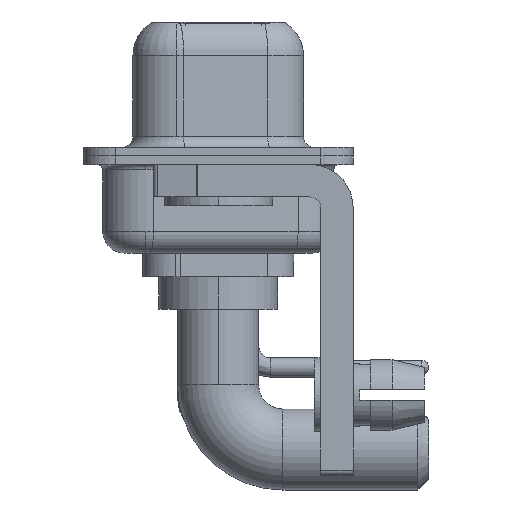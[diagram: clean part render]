
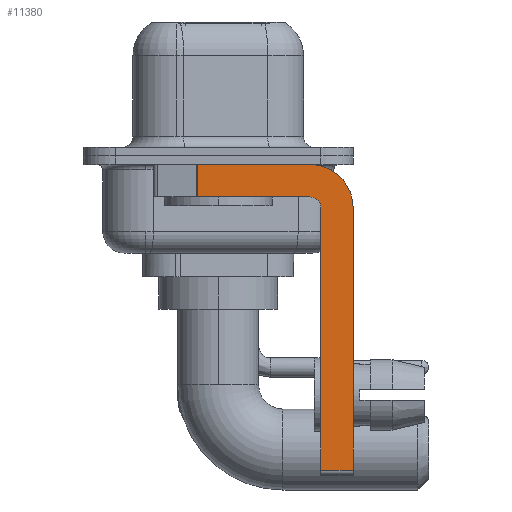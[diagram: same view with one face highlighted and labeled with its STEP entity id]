
A CAD part, left-side view. The second image highlights one B-rep face of the part: STEP entity #11380.
In plain terms, the highlighted planar face has unit normal (-1, 0, 0).
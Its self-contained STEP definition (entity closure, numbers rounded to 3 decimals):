
#782 = EDGE_CURVE ( 'NONE', #16685, #5322, #13096, .T. ) ;
#1770 = VERTEX_POINT ( 'NONE', #12619 ) ;
#1902 = VERTEX_POINT ( 'NONE', #8705 ) ;
#2012 = ORIENTED_EDGE ( 'NONE', *, *, #8583, .F. ) ;
#2090 = AXIS2_PLACEMENT_3D ( 'NONE', #5096, #18434, #12122 ) ;
#2623 = DIRECTION ( 'NONE',  ( 0., 0., -1. ) ) ;
#2792 = CIRCLE ( 'NONE', #18339, 2. ) ;
#2835 = LINE ( 'NONE', #13054, #6087 ) ;
#2849 = ORIENTED_EDGE ( 'NONE', *, *, #8291, .F. ) ;
#2997 = CARTESIAN_POINT ( 'NONE',  ( -2.9, -4.75, -14.8 ) ) ;
#3055 = DIRECTION ( 'NONE',  ( 0., 1., 0. ) ) ;
#3781 = LINE ( 'NONE', #16767, #17156 ) ;
#3980 = LINE ( 'NONE', #8471, #14771 ) ;
#4963 = LINE ( 'NONE', #6529, #10078 ) ;
#5096 = CARTESIAN_POINT ( 'NONE',  ( -2.9, -4.25, -2.4 ) ) ;
#5122 = EDGE_CURVE ( 'NONE', #1902, #5207, #3781, .T. ) ;
#5207 = VERTEX_POINT ( 'NONE', #18219 ) ;
#5322 = VERTEX_POINT ( 'NONE', #11475 ) ;
#6011 = DIRECTION ( 'NONE',  ( 0., 0., 1. ) ) ;
#6087 = VECTOR ( 'NONE', #10157, 1000. ) ;
#6529 = CARTESIAN_POINT ( 'NONE',  ( -2.9, 0.978, -1.9 ) ) ;
#6854 = EDGE_CURVE ( 'NONE', #12281, #7719, #4963, .T. ) ;
#7042 = ORIENTED_EDGE ( 'NONE', *, *, #6854, .T. ) ;
#7147 = CARTESIAN_POINT ( 'NONE',  ( -2.9, -4.25, -1.9 ) ) ;
#7312 = VERTEX_POINT ( 'NONE', #15230 ) ;
#7533 = ORIENTED_EDGE ( 'NONE', *, *, #14347, .F. ) ;
#7719 = VERTEX_POINT ( 'NONE', #13945 ) ;
#8124 = CARTESIAN_POINT ( 'NONE',  ( -2.9, -4.25, -2.4 ) ) ;
#8133 = FACE_OUTER_BOUND ( 'NONE', #12061, .T. ) ;
#8193 = DIRECTION ( 'NONE',  ( 0., -1., 0. ) ) ;
#8291 = EDGE_CURVE ( 'NONE', #12281, #7312, #3980, .T. ) ;
#8471 = CARTESIAN_POINT ( 'NONE',  ( -2.9, 3., -0.4 ) ) ;
#8583 = EDGE_CURVE ( 'NONE', #1770, #16685, #14673, .T. ) ;
#8705 = CARTESIAN_POINT ( 'NONE',  ( -2.9, -6.25, -2.4 ) ) ;
#9021 = ORIENTED_EDGE ( 'NONE', *, *, #17938, .T. ) ;
#9049 = AXIS2_PLACEMENT_3D ( 'NONE', #8124, #18234, #18334 ) ;
#9203 = VECTOR ( 'NONE', #6011, 1000. ) ;
#9953 = EDGE_CURVE ( 'NONE', #5322, #7719, #14827, .T. ) ;
#9958 = DIRECTION ( 'NONE',  ( 1., 0., 0. ) ) ;
#10078 = VECTOR ( 'NONE', #16835, 1000. ) ;
#10157 = DIRECTION ( 'NONE',  ( 0., -1., 0. ) ) ;
#11201 = CARTESIAN_POINT ( 'NONE',  ( -2.9, 0.978, -0.4 ) ) ;
#11380 = ADVANCED_FACE ( 'NONE', ( #8133 ), #12310, .F. ) ;
#11475 = CARTESIAN_POINT ( 'NONE',  ( -2.9, -4.25, -1.9 ) ) ;
#12061 = EDGE_LOOP ( 'NONE', ( #2849, #7042, #18802, #12797, #2012, #9021, #13911, #7533 ) ) ;
#12122 = DIRECTION ( 'NONE',  ( 0., 0., -1. ) ) ;
#12224 = CARTESIAN_POINT ( 'NONE',  ( -2.9, -4.75, -2.4 ) ) ;
#12281 = VERTEX_POINT ( 'NONE', #11201 ) ;
#12310 = PLANE ( 'NONE',  #2090 ) ;
#12619 = CARTESIAN_POINT ( 'NONE',  ( -2.9, -4.75, -14.55 ) ) ;
#12797 = ORIENTED_EDGE ( 'NONE', *, *, #782, .F. ) ;
#13054 = CARTESIAN_POINT ( 'NONE',  ( -2.9, -4.25, -14.55 ) ) ;
#13096 = CIRCLE ( 'NONE', #9049, 0.5 ) ;
#13911 = ORIENTED_EDGE ( 'NONE', *, *, #5122, .F. ) ;
#13945 = CARTESIAN_POINT ( 'NONE',  ( -2.9, 0.978, -1.9 ) ) ;
#14347 = EDGE_CURVE ( 'NONE', #7312, #1902, #2792, .T. ) ;
#14673 = LINE ( 'NONE', #2997, #9203 ) ;
#14771 = VECTOR ( 'NONE', #8193, 1000. ) ;
#14827 = LINE ( 'NONE', #7147, #17632 ) ;
#15230 = CARTESIAN_POINT ( 'NONE',  ( -2.9, -4.25, -0.4 ) ) ;
#16685 = VERTEX_POINT ( 'NONE', #12224 ) ;
#16767 = CARTESIAN_POINT ( 'NONE',  ( -2.9, -6.25, -2.4 ) ) ;
#16835 = DIRECTION ( 'NONE',  ( 0., 0., -1. ) ) ;
#17156 = VECTOR ( 'NONE', #18120, 1000. ) ;
#17244 = CARTESIAN_POINT ( 'NONE',  ( -2.9, -4.25, -2.4 ) ) ;
#17632 = VECTOR ( 'NONE', #3055, 1000. ) ;
#17938 = EDGE_CURVE ( 'NONE', #1770, #5207, #2835, .T. ) ;
#18120 = DIRECTION ( 'NONE',  ( 0., 0., -1. ) ) ;
#18219 = CARTESIAN_POINT ( 'NONE',  ( -2.9, -6.25, -14.55 ) ) ;
#18234 = DIRECTION ( 'NONE',  ( -1., 0., 0. ) ) ;
#18334 = DIRECTION ( 'NONE',  ( 0., 0., 1. ) ) ;
#18339 = AXIS2_PLACEMENT_3D ( 'NONE', #17244, #9958, #2623 ) ;
#18434 = DIRECTION ( 'NONE',  ( 1., 0., 0. ) ) ;
#18802 = ORIENTED_EDGE ( 'NONE', *, *, #9953, .F. ) ;
